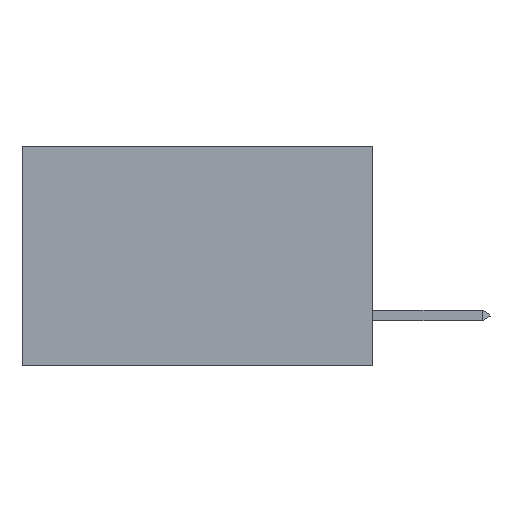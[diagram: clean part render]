
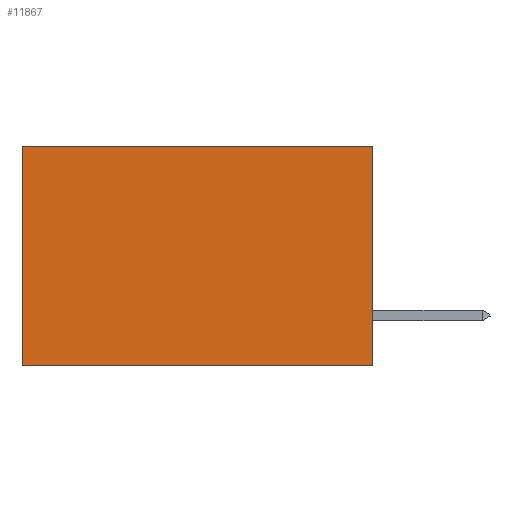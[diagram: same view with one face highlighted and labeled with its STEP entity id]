
A CAD part, left-side view. The second image highlights one B-rep face of the part: STEP entity #11867.
In plain terms, the highlighted planar face has unit normal (-1, 0, 0).
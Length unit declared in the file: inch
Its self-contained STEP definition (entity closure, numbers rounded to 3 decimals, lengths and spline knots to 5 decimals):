
#1728 = LINE ( 'NONE', #26366, #13567 ) ;
#2301 = CARTESIAN_POINT ( 'NONE',  ( 0.277, 0., -0.37 ) ) ;
#3302 = PLANE ( 'NONE',  #7459 ) ;
#3620 = VERTEX_POINT ( 'NONE', #28403 ) ;
#3726 = EDGE_CURVE ( 'NONE', #7350, #3620, #17016, .T. ) ;
#4701 = DIRECTION ( 'NONE',  ( 0., 0., -1. ) ) ;
#4753 = VECTOR ( 'NONE', #24648, 39.37008 ) ;
#5838 = ORIENTED_EDGE ( 'NONE', *, *, #13721, .T. ) ;
#7350 = VERTEX_POINT ( 'NONE', #20099 ) ;
#7459 = AXIS2_PLACEMENT_3D ( 'NONE', #15057, #8103, #24565 ) ;
#8103 = DIRECTION ( 'NONE',  ( 1., 0., 0. ) ) ;
#9135 = DIRECTION ( 'NONE',  ( 0., 0., -1. ) ) ;
#10807 = VECTOR ( 'NONE', #9135, 39.37008 ) ;
#11867 = ADVANCED_FACE ( 'NONE', ( #15537 ), #3302, .F. ) ;
#12247 = VERTEX_POINT ( 'NONE', #21095 ) ;
#13567 = VECTOR ( 'NONE', #14451, 39.37008 ) ;
#13721 = EDGE_CURVE ( 'NONE', #18394, #7350, #1728, .T. ) ;
#14451 = DIRECTION ( 'NONE',  ( 0., 1., 0. ) ) ;
#15057 = CARTESIAN_POINT ( 'NONE',  ( 0.277, 0., -0.37 ) ) ;
#15537 = FACE_OUTER_BOUND ( 'NONE', #23819, .T. ) ;
#15818 = CARTESIAN_POINT ( 'NONE',  ( 0.277, 0., 0. ) ) ;
#16145 = ORIENTED_EDGE ( 'NONE', *, *, #3726, .T. ) ;
#17016 = LINE ( 'NONE', #23200, #10807 ) ;
#18394 = VERTEX_POINT ( 'NONE', #15818 ) ;
#18536 = EDGE_CURVE ( 'NONE', #18394, #12247, #21780, .T. ) ;
#20099 = CARTESIAN_POINT ( 'NONE',  ( 0.277, 0.59, 0. ) ) ;
#21095 = CARTESIAN_POINT ( 'NONE',  ( 0.277, 0., -0.37 ) ) ;
#21780 = LINE ( 'NONE', #2301, #27447 ) ;
#22234 = CARTESIAN_POINT ( 'NONE',  ( 0.277, 0., -0.37 ) ) ;
#22381 = ORIENTED_EDGE ( 'NONE', *, *, #24901, .F. ) ;
#23200 = CARTESIAN_POINT ( 'NONE',  ( 0.277, 0.59, -0.37 ) ) ;
#23507 = LINE ( 'NONE', #22234, #4753 ) ;
#23819 = EDGE_LOOP ( 'NONE', ( #16145, #22381, #30282, #5838 ) ) ;
#24565 = DIRECTION ( 'NONE',  ( 0., 0., -1. ) ) ;
#24648 = DIRECTION ( 'NONE',  ( 0., 1., 0. ) ) ;
#24901 = EDGE_CURVE ( 'NONE', #12247, #3620, #23507, .T. ) ;
#26366 = CARTESIAN_POINT ( 'NONE',  ( 0.277, 0., 0. ) ) ;
#27447 = VECTOR ( 'NONE', #4701, 39.37008 ) ;
#28403 = CARTESIAN_POINT ( 'NONE',  ( 0.277, 0.59, -0.37 ) ) ;
#30282 = ORIENTED_EDGE ( 'NONE', *, *, #18536, .F. ) ;
